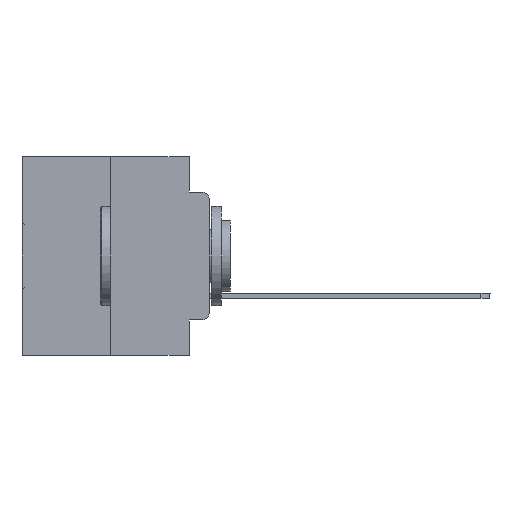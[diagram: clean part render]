
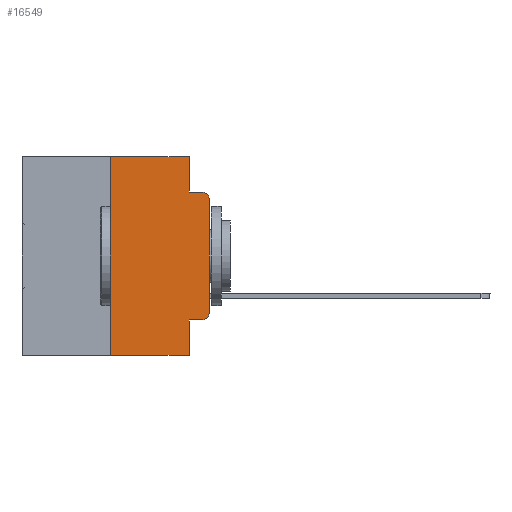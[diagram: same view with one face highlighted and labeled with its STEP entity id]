
A CAD part, left-side view. The second image highlights one B-rep face of the part: STEP entity #16549.
In plain terms, the highlighted planar face has unit normal (-1, 0, 0).
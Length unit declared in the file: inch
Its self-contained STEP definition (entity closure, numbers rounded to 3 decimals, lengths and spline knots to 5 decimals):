
#204 = ORIENTED_EDGE ( 'NONE', *, *, #19435, .T. ) ;
#1168 = ORIENTED_EDGE ( 'NONE', *, *, #30485, .F. ) ;
#1193 = LINE ( 'NONE', #28776, #32255 ) ;
#1463 = VECTOR ( 'NONE', #11017, 39.37008 ) ;
#2233 = EDGE_CURVE ( 'NONE', #10525, #7215, #1193, .T. ) ;
#2299 = VERTEX_POINT ( 'NONE', #6162 ) ;
#2312 = EDGE_CURVE ( 'NONE', #25678, #9207, #26778, .T. ) ;
#3805 = VECTOR ( 'NONE', #11908, 39.37008 ) ;
#3864 = VECTOR ( 'NONE', #27716, 39.37008 ) ;
#4804 = CARTESIAN_POINT ( 'NONE',  ( 0., 0.051, 0. ) ) ;
#5411 = LINE ( 'NONE', #9861, #8725 ) ;
#5931 = LINE ( 'NONE', #28866, #22975 ) ;
#6162 = CARTESIAN_POINT ( 'NONE',  ( 0., 0.051, -0.5 ) ) ;
#6188 = CARTESIAN_POINT ( 'NONE',  ( 0., 0.25, 0. ) ) ;
#6639 = CARTESIAN_POINT ( 'NONE',  ( 0., 0.25, 0. ) ) ;
#6703 = VERTEX_POINT ( 'NONE', #29002 ) ;
#7215 = VERTEX_POINT ( 'NONE', #24644 ) ;
#7607 = FACE_OUTER_BOUND ( 'NONE', #9768, .T. ) ;
#7817 = CARTESIAN_POINT ( 'NONE',  ( 0., 0.02, -0.0885 ) ) ;
#8405 = DIRECTION ( 'NONE',  ( 0., 0., -1. ) ) ;
#8725 = VECTOR ( 'NONE', #12845, 39.37008 ) ;
#9207 = VERTEX_POINT ( 'NONE', #6188 ) ;
#9319 = CARTESIAN_POINT ( 'NONE',  ( 0., 0.02, -0.1085 ) ) ;
#9434 = VERTEX_POINT ( 'NONE', #7817 ) ;
#9768 = EDGE_LOOP ( 'NONE', ( #16422, #27379, #13338, #11605, #25738, #24322, #10041, #1168, #204, #23815 ) ) ;
#9861 = CARTESIAN_POINT ( 'NONE',  ( 0., 0.473, 0. ) ) ;
#10041 = ORIENTED_EDGE ( 'NONE', *, *, #25152, .T. ) ;
#10525 = VERTEX_POINT ( 'NONE', #11942 ) ;
#10538 = LINE ( 'NONE', #31008, #1463 ) ;
#11017 = DIRECTION ( 'NONE',  ( 0., -1., 0. ) ) ;
#11164 = CARTESIAN_POINT ( 'NONE',  ( 0., 0.02, -0.4115 ) ) ;
#11268 = DIRECTION ( 'NONE',  ( 0., 0., 1. ) ) ;
#11526 = VECTOR ( 'NONE', #22191, 39.37008 ) ;
#11605 = ORIENTED_EDGE ( 'NONE', *, *, #30979, .F. ) ;
#11627 = AXIS2_PLACEMENT_3D ( 'NONE', #24939, #12392, #27570 ) ;
#11908 = DIRECTION ( 'NONE',  ( 0., 0., 1. ) ) ;
#11942 = CARTESIAN_POINT ( 'NONE',  ( 0., 0., -0.3915 ) ) ;
#12200 = DIRECTION ( 'NONE',  ( 0., 0., -1. ) ) ;
#12392 = DIRECTION ( 'NONE',  ( 1., 0., 0. ) ) ;
#12434 = VECTOR ( 'NONE', #16540, 39.37008 ) ;
#12585 = CARTESIAN_POINT ( 'NONE',  ( 0., 0.051, -0.4115 ) ) ;
#12845 = DIRECTION ( 'NONE',  ( 0., -1., 0. ) ) ;
#13338 = ORIENTED_EDGE ( 'NONE', *, *, #27191, .F. ) ;
#13762 = LINE ( 'NONE', #31411, #12434 ) ;
#14765 = LINE ( 'NONE', #29632, #11526 ) ;
#14859 = PLANE ( 'NONE',  #11627 ) ;
#14896 = VERTEX_POINT ( 'NONE', #11164 ) ;
#15001 = CARTESIAN_POINT ( 'NONE',  ( 0., 0.051, -0.4115 ) ) ;
#16422 = ORIENTED_EDGE ( 'NONE', *, *, #2233, .T. ) ;
#16540 = DIRECTION ( 'NONE',  ( 0., 0., -1. ) ) ;
#16549 = ADVANCED_FACE ( 'NONE', ( #7607 ), #14859, .F. ) ;
#16563 = AXIS2_PLACEMENT_3D ( 'NONE', #9319, #32591, #22356 ) ;
#17649 = LINE ( 'NONE', #15001, #3864 ) ;
#18152 = CIRCLE ( 'NONE', #16563, 0.02 ) ;
#19435 = EDGE_CURVE ( 'NONE', #27565, #14896, #17649, .T. ) ;
#20505 = CIRCLE ( 'NONE', #23688, 0.02 ) ;
#22191 = DIRECTION ( 'NONE',  ( 0., -1., 0. ) ) ;
#22356 = DIRECTION ( 'NONE',  ( 0., 0., -1. ) ) ;
#22897 = EDGE_CURVE ( 'NONE', #9207, #28923, #5411, .T. ) ;
#22975 = VECTOR ( 'NONE', #8405, 39.37008 ) ;
#23688 = AXIS2_PLACEMENT_3D ( 'NONE', #26565, #29545, #12200 ) ;
#23815 = ORIENTED_EDGE ( 'NONE', *, *, #26122, .T. ) ;
#24322 = ORIENTED_EDGE ( 'NONE', *, *, #2312, .F. ) ;
#24644 = CARTESIAN_POINT ( 'NONE',  ( 0., 0., -0.1085 ) ) ;
#24939 = CARTESIAN_POINT ( 'NONE',  ( 0., 0.473, 0. ) ) ;
#25152 = EDGE_CURVE ( 'NONE', #25678, #2299, #10538, .T. ) ;
#25678 = VERTEX_POINT ( 'NONE', #31274 ) ;
#25738 = ORIENTED_EDGE ( 'NONE', *, *, #22897, .F. ) ;
#26122 = EDGE_CURVE ( 'NONE', #14896, #10525, #20505, .T. ) ;
#26565 = CARTESIAN_POINT ( 'NONE',  ( 0., 0.02, -0.3915 ) ) ;
#26778 = LINE ( 'NONE', #6639, #3805 ) ;
#27191 = EDGE_CURVE ( 'NONE', #6703, #9434, #14765, .T. ) ;
#27379 = ORIENTED_EDGE ( 'NONE', *, *, #29671, .T. ) ;
#27565 = VERTEX_POINT ( 'NONE', #12585 ) ;
#27570 = DIRECTION ( 'NONE',  ( 0., 0., -1. ) ) ;
#27716 = DIRECTION ( 'NONE',  ( 0., -1., 0. ) ) ;
#28776 = CARTESIAN_POINT ( 'NONE',  ( 0., 0., 0. ) ) ;
#28866 = CARTESIAN_POINT ( 'NONE',  ( 0., 0.051, 0. ) ) ;
#28923 = VERTEX_POINT ( 'NONE', #4804 ) ;
#29002 = CARTESIAN_POINT ( 'NONE',  ( 0., 0.051, -0.0885 ) ) ;
#29545 = DIRECTION ( 'NONE',  ( -1., 0., 0. ) ) ;
#29632 = CARTESIAN_POINT ( 'NONE',  ( 0., 0.051, -0.0885 ) ) ;
#29671 = EDGE_CURVE ( 'NONE', #7215, #9434, #18152, .T. ) ;
#30485 = EDGE_CURVE ( 'NONE', #27565, #2299, #5931, .T. ) ;
#30979 = EDGE_CURVE ( 'NONE', #28923, #6703, #13762, .T. ) ;
#31008 = CARTESIAN_POINT ( 'NONE',  ( 0., 0.473, -0.5 ) ) ;
#31274 = CARTESIAN_POINT ( 'NONE',  ( 0., 0.25, -0.5 ) ) ;
#31411 = CARTESIAN_POINT ( 'NONE',  ( 0., 0.051, 0. ) ) ;
#32255 = VECTOR ( 'NONE', #11268, 39.37008 ) ;
#32591 = DIRECTION ( 'NONE',  ( -1., 0., 0. ) ) ;
